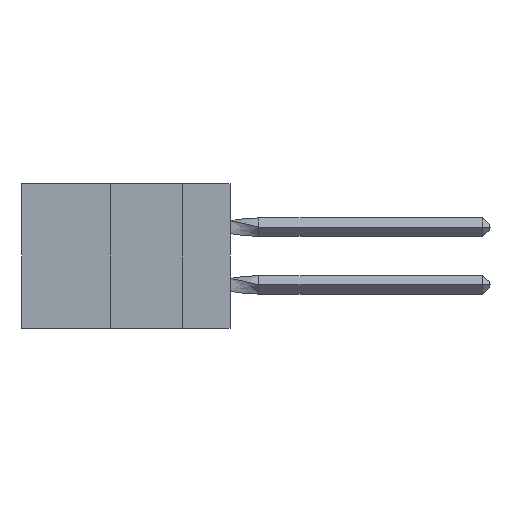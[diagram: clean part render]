
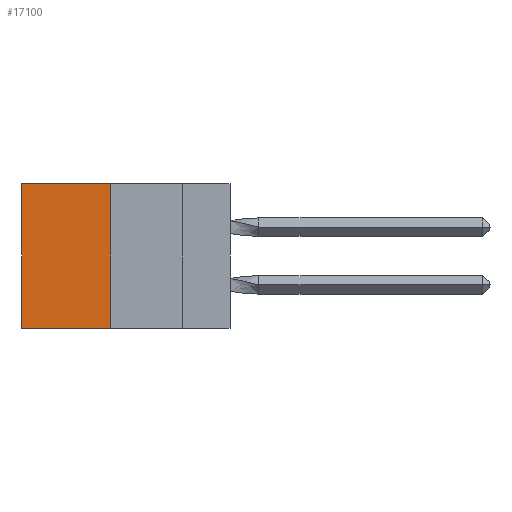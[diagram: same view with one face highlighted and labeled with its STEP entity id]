
A CAD part, left-side view. The second image highlights one B-rep face of the part: STEP entity #17100.
In plain terms, the highlighted planar face has unit normal (-1, 0, 0).
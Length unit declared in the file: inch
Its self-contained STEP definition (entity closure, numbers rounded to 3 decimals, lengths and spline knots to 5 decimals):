
#357 = EDGE_CURVE ( 'NONE', #33355, #16227, #22741, .T. ) ;
#450 = EDGE_CURVE ( 'NONE', #23778, #16227, #25880, .T. ) ;
#828 = DIRECTION ( 'NONE',  ( 0., 0., -1. ) ) ;
#878 = LINE ( 'NONE', #23231, #30544 ) ;
#1123 = EDGE_LOOP ( 'NONE', ( #8997, #15230, #23705, #25222 ) ) ;
#3470 = CARTESIAN_POINT ( 'NONE',  ( 0.305, 0.72, -0.5 ) ) ;
#4398 = CARTESIAN_POINT ( 'NONE',  ( 0.305, 0.413, 0. ) ) ;
#7403 = DIRECTION ( 'NONE',  ( 0., 0., -1. ) ) ;
#8453 = EDGE_CURVE ( 'NONE', #24155, #23778, #18497, .T. ) ;
#8997 = ORIENTED_EDGE ( 'NONE', *, *, #357, .T. ) ;
#9131 = FACE_OUTER_BOUND ( 'NONE', #1123, .T. ) ;
#9575 = VECTOR ( 'NONE', #7403, 39.37008 ) ;
#10010 = EDGE_CURVE ( 'NONE', #24155, #33355, #878, .T. ) ;
#12452 = VECTOR ( 'NONE', #21675, 39.37008 ) ;
#15059 = CARTESIAN_POINT ( 'NONE',  ( 0.305, 0.413, -0.5 ) ) ;
#15184 = DIRECTION ( 'NONE',  ( 1., 0., 0. ) ) ;
#15230 = ORIENTED_EDGE ( 'NONE', *, *, #450, .F. ) ;
#16227 = VERTEX_POINT ( 'NONE', #3470 ) ;
#17100 = ADVANCED_FACE ( 'NONE', ( #9131 ), #32142, .F. ) ;
#18497 = LINE ( 'NONE', #36131, #9575 ) ;
#19022 = CARTESIAN_POINT ( 'NONE',  ( 0.305, 0.72, -0.5 ) ) ;
#21675 = DIRECTION ( 'NONE',  ( 0., 0., -1. ) ) ;
#22122 = CARTESIAN_POINT ( 'NONE',  ( 0.305, 0.413, -0.5 ) ) ;
#22741 = LINE ( 'NONE', #19022, #12452 ) ;
#23231 = CARTESIAN_POINT ( 'NONE',  ( 0.305, 0.413, 0. ) ) ;
#23705 = ORIENTED_EDGE ( 'NONE', *, *, #8453, .F. ) ;
#23778 = VERTEX_POINT ( 'NONE', #22122 ) ;
#24005 = AXIS2_PLACEMENT_3D ( 'NONE', #15059, #15184, #828 ) ;
#24155 = VERTEX_POINT ( 'NONE', #4398 ) ;
#25222 = ORIENTED_EDGE ( 'NONE', *, *, #10010, .T. ) ;
#25880 = LINE ( 'NONE', #30692, #34423 ) ;
#26100 = DIRECTION ( 'NONE',  ( 0., 1., 0. ) ) ;
#27909 = DIRECTION ( 'NONE',  ( 0., 1., 0. ) ) ;
#30544 = VECTOR ( 'NONE', #26100, 39.37008 ) ;
#30692 = CARTESIAN_POINT ( 'NONE',  ( 0.305, 0.413, -0.5 ) ) ;
#32142 = PLANE ( 'NONE',  #24005 ) ;
#33355 = VERTEX_POINT ( 'NONE', #33799 ) ;
#33799 = CARTESIAN_POINT ( 'NONE',  ( 0.305, 0.72, 0. ) ) ;
#34423 = VECTOR ( 'NONE', #27909, 39.37008 ) ;
#36131 = CARTESIAN_POINT ( 'NONE',  ( 0.305, 0.413, -0.5 ) ) ;
